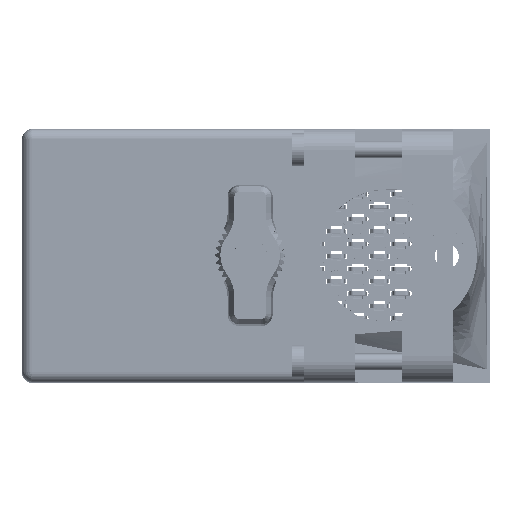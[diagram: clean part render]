
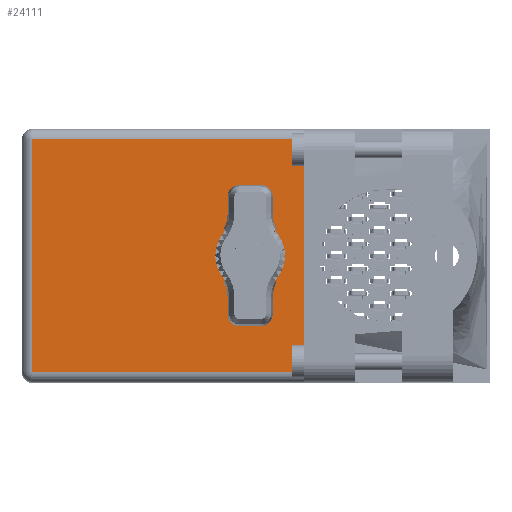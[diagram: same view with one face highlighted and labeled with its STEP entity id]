
A CAD part, top view. The second image highlights one B-rep face of the part: STEP entity #24111.
In plain terms, the highlighted face is planar.
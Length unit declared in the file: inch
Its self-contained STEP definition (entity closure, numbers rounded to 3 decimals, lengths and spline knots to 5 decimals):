
#1250 = ORIENTED_EDGE ( 'NONE', *, *, #95665, .F. ) ;
#5693 = VERTEX_POINT ( 'NONE', #59727 ) ;
#7427 = VERTEX_POINT ( 'NONE', #103718 ) ;
#13620 = DIRECTION ( 'NONE',  ( 1., 0., 0. ) ) ;
#16331 = CARTESIAN_POINT ( 'NONE',  ( -1.3155, 1.93, -0.765 ) ) ;
#18267 = DIRECTION ( 'NONE',  ( 0., 0., 1. ) ) ;
#19063 = DIRECTION ( 'NONE',  ( -1., 0., 0. ) ) ;
#19719 = EDGE_CURVE ( 'NONE', #7427, #55313, #52795, .T. ) ;
#21473 = VECTOR ( 'NONE', #96661, 39.37008 ) ;
#24111 = ADVANCED_FACE ( 'NONE', ( #96017, #103545 ), #62828, .T. ) ;
#24680 = CARTESIAN_POINT ( 'NONE',  ( -1.3155, 1.93, -0.703 ) ) ;
#24778 = VECTOR ( 'NONE', #13620, 39.37008 ) ;
#26131 = EDGE_CURVE ( 'NONE', #66533, #5693, #38554, .T. ) ;
#26310 = CARTESIAN_POINT ( 'NONE',  ( 0., 1.93, 0. ) ) ;
#27839 = DIRECTION ( 'NONE',  ( 0., 1., 0. ) ) ;
#28518 = ORIENTED_EDGE ( 'NONE', *, *, #68621, .F. ) ;
#38554 = CIRCLE ( 'NONE', #64238, 0.17 ) ;
#39296 = LINE ( 'NONE', #87001, #24778 ) ;
#41378 = DIRECTION ( 'NONE',  ( 0., 0., 1. ) ) ;
#41674 = CARTESIAN_POINT ( 'NONE',  ( -1.3155, 1.93, 0.703 ) ) ;
#51414 = EDGE_CURVE ( 'NONE', #55313, #87859, #98773, .T. ) ;
#51530 = CARTESIAN_POINT ( 'NONE',  ( 0.3275, 1.93, -0.765 ) ) ;
#52795 = LINE ( 'NONE', #92428, #80628 ) ;
#55313 = VERTEX_POINT ( 'NONE', #24680 ) ;
#55395 = AXIS2_PLACEMENT_3D ( 'NONE', #77858, #61250, #95487 ) ;
#59727 = CARTESIAN_POINT ( 'NONE',  ( 0., 1.93, 0.17 ) ) ;
#60458 = ORIENTED_EDGE ( 'NONE', *, *, #19719, .T. ) ;
#61119 = EDGE_LOOP ( 'NONE', ( #70792, #69322, #1250, #60458 ) ) ;
#61250 = DIRECTION ( 'NONE',  ( 0., 1., 0. ) ) ;
#62828 = PLANE ( 'NONE',  #55395 ) ;
#64238 = AXIS2_PLACEMENT_3D ( 'NONE', #66947, #27839, #74473 ) ;
#66337 = CARTESIAN_POINT ( 'NONE',  ( 0.3275, 1.93, 0.703 ) ) ;
#66533 = VERTEX_POINT ( 'NONE', #98748 ) ;
#66947 = CARTESIAN_POINT ( 'NONE',  ( 0., 1.93, 0. ) ) ;
#68621 = EDGE_CURVE ( 'NONE', #5693, #66533, #91261, .T. ) ;
#69322 = ORIENTED_EDGE ( 'NONE', *, *, #104432, .T. ) ;
#70792 = ORIENTED_EDGE ( 'NONE', *, *, #51414, .T. ) ;
#73435 = EDGE_LOOP ( 'NONE', ( #28518, #89156 ) ) ;
#74473 = DIRECTION ( 'NONE',  ( 0., 0., 1. ) ) ;
#75580 = DIRECTION ( 'NONE',  ( 0., 1., 0. ) ) ;
#77858 = CARTESIAN_POINT ( 'NONE',  ( -1.3775, 1.93, -0.765 ) ) ;
#80628 = VECTOR ( 'NONE', #19063, 39.37008 ) ;
#84396 = AXIS2_PLACEMENT_3D ( 'NONE', #26310, #75580, #18267 ) ;
#85929 = VERTEX_POINT ( 'NONE', #66337 ) ;
#87001 = CARTESIAN_POINT ( 'NONE',  ( 0.3275, 1.93, 0.703 ) ) ;
#87859 = VERTEX_POINT ( 'NONE', #41674 ) ;
#89156 = ORIENTED_EDGE ( 'NONE', *, *, #26131, .F. ) ;
#90651 = LINE ( 'NONE', #51530, #97176 ) ;
#91261 = CIRCLE ( 'NONE', #84396, 0.17 ) ;
#92428 = CARTESIAN_POINT ( 'NONE',  ( -1.3775, 1.93, -0.703 ) ) ;
#95487 = DIRECTION ( 'NONE',  ( -1., 0., 0. ) ) ;
#95665 = EDGE_CURVE ( 'NONE', #7427, #85929, #90651, .T. ) ;
#96017 = FACE_OUTER_BOUND ( 'NONE', #61119, .T. ) ;
#96661 = DIRECTION ( 'NONE',  ( 0., 0., 1. ) ) ;
#97176 = VECTOR ( 'NONE', #41378, 39.37008 ) ;
#98748 = CARTESIAN_POINT ( 'NONE',  ( 0., 1.93, -0.17 ) ) ;
#98773 = LINE ( 'NONE', #16331, #21473 ) ;
#103545 = FACE_BOUND ( 'NONE', #73435, .T. ) ;
#103718 = CARTESIAN_POINT ( 'NONE',  ( 0.3275, 1.93, -0.703 ) ) ;
#104432 = EDGE_CURVE ( 'NONE', #87859, #85929, #39296, .T. ) ;
